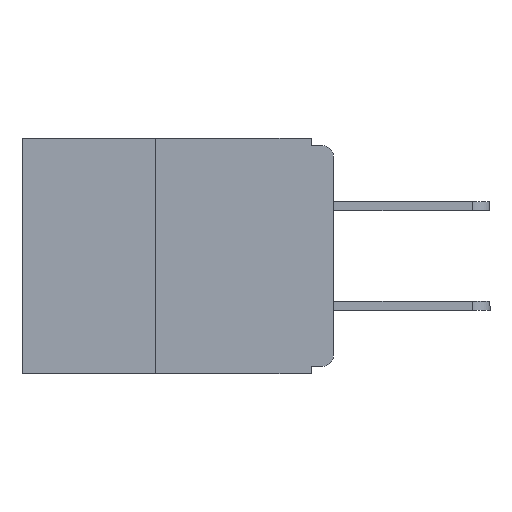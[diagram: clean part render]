
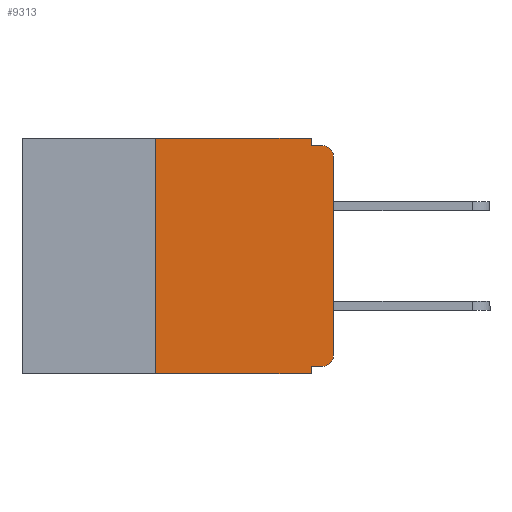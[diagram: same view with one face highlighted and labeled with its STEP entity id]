
A CAD part, left-side view. The second image highlights one B-rep face of the part: STEP entity #9313.
In plain terms, the highlighted planar face has unit normal (-1, 0, 0).
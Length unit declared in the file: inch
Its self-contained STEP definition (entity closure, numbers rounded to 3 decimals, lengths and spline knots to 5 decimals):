
#285 = VERTEX_POINT ( 'NONE', #8248 ) ;
#560 = VECTOR ( 'NONE', #4195, 39.37008 ) ;
#679 = DIRECTION ( 'NONE',  ( 0., 0., 1. ) ) ;
#684 = VERTEX_POINT ( 'NONE', #11078 ) ;
#914 = LINE ( 'NONE', #20379, #15717 ) ;
#1093 = VECTOR ( 'NONE', #679, 39.37008 ) ;
#1956 = DIRECTION ( 'NONE',  ( 1., 0., 0. ) ) ;
#2394 = DIRECTION ( 'NONE',  ( -1., 0., 0. ) ) ;
#2707 = EDGE_CURVE ( 'NONE', #684, #4057, #21120, .T. ) ;
#3035 = CARTESIAN_POINT ( 'NONE',  ( 0., 0.25, 0. ) ) ;
#3144 = CARTESIAN_POINT ( 'NONE',  ( 0., 0.031, -0.32 ) ) ;
#3458 = VERTEX_POINT ( 'NONE', #3035 ) ;
#3592 = PLANE ( 'NONE',  #4601 ) ;
#4008 = EDGE_LOOP ( 'NONE', ( #6687, #7054, #7076, #7227, #7481, #7824, #8143, #8163, #8323, #8462 ) ) ;
#4057 = VERTEX_POINT ( 'NONE', #13959 ) ;
#4117 = LINE ( 'NONE', #20929, #13785 ) ;
#4195 = DIRECTION ( 'NONE',  ( 0., 1., 0. ) ) ;
#4463 = CIRCLE ( 'NONE', #12592, 0.015 ) ;
#4500 = AXIS2_PLACEMENT_3D ( 'NONE', #12736, #2394, #14424 ) ;
#4601 = AXIS2_PLACEMENT_3D ( 'NONE', #5316, #1956, #21097 ) ;
#4613 = DIRECTION ( 'NONE',  ( -1., 0., 0. ) ) ;
#4679 = LINE ( 'NONE', #7680, #560 ) ;
#5316 = CARTESIAN_POINT ( 'NONE',  ( 0., 0.437, 0. ) ) ;
#5976 = VECTOR ( 'NONE', #12562, 39.37008 ) ;
#6687 = ORIENTED_EDGE ( 'NONE', *, *, #2707, .T. ) ;
#7054 = ORIENTED_EDGE ( 'NONE', *, *, #12635, .T. ) ;
#7076 = ORIENTED_EDGE ( 'NONE', *, *, #15427, .F. ) ;
#7227 = ORIENTED_EDGE ( 'NONE', *, *, #19667, .F. ) ;
#7481 = ORIENTED_EDGE ( 'NONE', *, *, #15186, .F. ) ;
#7680 = CARTESIAN_POINT ( 'NONE',  ( 0., 0., -0.32 ) ) ;
#7824 = ORIENTED_EDGE ( 'NONE', *, *, #20200, .F. ) ;
#8143 = ORIENTED_EDGE ( 'NONE', *, *, #9243, .T. ) ;
#8163 = ORIENTED_EDGE ( 'NONE', *, *, #12153, .F. ) ;
#8248 = CARTESIAN_POINT ( 'NONE',  ( 0., 0.015, -0.32 ) ) ;
#8323 = ORIENTED_EDGE ( 'NONE', *, *, #13721, .F. ) ;
#8462 = ORIENTED_EDGE ( 'NONE', *, *, #18484, .T. ) ;
#9059 = VERTEX_POINT ( 'NONE', #9771 ) ;
#9243 = EDGE_CURVE ( 'NONE', #19841, #9059, #17347, .T. ) ;
#9313 = ADVANCED_FACE ( 'NONE', ( #15789 ), #3592, .F. ) ;
#9710 = VECTOR ( 'NONE', #11576, 39.37008 ) ;
#9771 = CARTESIAN_POINT ( 'NONE',  ( 0., 0.031, -0.33 ) ) ;
#9897 = CARTESIAN_POINT ( 'NONE',  ( 0., 0.25, -0.33 ) ) ;
#10280 = LINE ( 'NONE', #14981, #9710 ) ;
#10506 = DIRECTION ( 'NONE',  ( 0., 0., -1. ) ) ;
#11077 = CARTESIAN_POINT ( 'NONE',  ( 0., 0.25, -0.33 ) ) ;
#11078 = CARTESIAN_POINT ( 'NONE',  ( 0., 0., -0.305 ) ) ;
#11576 = DIRECTION ( 'NONE',  ( 0., -1., 0. ) ) ;
#11728 = CARTESIAN_POINT ( 'NONE',  ( 0., 0.031, -0.01 ) ) ;
#12050 = CARTESIAN_POINT ( 'NONE',  ( 0., 0.437, -0.33 ) ) ;
#12153 = EDGE_CURVE ( 'NONE', #13985, #9059, #914, .T. ) ;
#12394 = VECTOR ( 'NONE', #21796, 39.37008 ) ;
#12462 = VECTOR ( 'NONE', #16134, 39.37008 ) ;
#12562 = DIRECTION ( 'NONE',  ( 0., -1., 0. ) ) ;
#12592 = AXIS2_PLACEMENT_3D ( 'NONE', #14888, #4613, #16549 ) ;
#12635 = EDGE_CURVE ( 'NONE', #4057, #15922, #4463, .T. ) ;
#12736 = CARTESIAN_POINT ( 'NONE',  ( 0., 0.015, -0.305 ) ) ;
#12834 = DIRECTION ( 'NONE',  ( 0., 0., -1. ) ) ;
#13721 = EDGE_CURVE ( 'NONE', #285, #13985, #4679, .T. ) ;
#13785 = VECTOR ( 'NONE', #12834, 39.37008 ) ;
#13959 = CARTESIAN_POINT ( 'NONE',  ( 0., 0., -0.025 ) ) ;
#13985 = VERTEX_POINT ( 'NONE', #3144 ) ;
#13996 = VERTEX_POINT ( 'NONE', #11728 ) ;
#14324 = LINE ( 'NONE', #11077, #1093 ) ;
#14424 = DIRECTION ( 'NONE',  ( 0., 0., -1. ) ) ;
#14888 = CARTESIAN_POINT ( 'NONE',  ( 0., 0.015, -0.025 ) ) ;
#14981 = CARTESIAN_POINT ( 'NONE',  ( 0., 0., -0.01 ) ) ;
#15186 = EDGE_CURVE ( 'NONE', #3458, #16018, #19866, .T. ) ;
#15427 = EDGE_CURVE ( 'NONE', #13996, #15922, #10280, .T. ) ;
#15717 = VECTOR ( 'NONE', #10506, 39.37008 ) ;
#15789 = FACE_OUTER_BOUND ( 'NONE', #4008, .T. ) ;
#15848 = CARTESIAN_POINT ( 'NONE',  ( 0., 0.437, 0. ) ) ;
#15922 = VERTEX_POINT ( 'NONE', #21063 ) ;
#16018 = VERTEX_POINT ( 'NONE', #18141 ) ;
#16134 = DIRECTION ( 'NONE',  ( 0., 0., 1. ) ) ;
#16153 = CARTESIAN_POINT ( 'NONE',  ( 0., 0., 0. ) ) ;
#16549 = DIRECTION ( 'NONE',  ( 0., 0., -1. ) ) ;
#17347 = LINE ( 'NONE', #12050, #12394 ) ;
#18141 = CARTESIAN_POINT ( 'NONE',  ( 0., 0.031, 0. ) ) ;
#18484 = EDGE_CURVE ( 'NONE', #285, #684, #20442, .T. ) ;
#19667 = EDGE_CURVE ( 'NONE', #16018, #13996, #4117, .T. ) ;
#19841 = VERTEX_POINT ( 'NONE', #9897 ) ;
#19866 = LINE ( 'NONE', #15848, #5976 ) ;
#20200 = EDGE_CURVE ( 'NONE', #19841, #3458, #14324, .T. ) ;
#20379 = CARTESIAN_POINT ( 'NONE',  ( 0., 0.031, -0.33 ) ) ;
#20442 = CIRCLE ( 'NONE', #4500, 0.015 ) ;
#20929 = CARTESIAN_POINT ( 'NONE',  ( 0., 0.031, 0. ) ) ;
#21063 = CARTESIAN_POINT ( 'NONE',  ( 0., 0.015, -0.01 ) ) ;
#21097 = DIRECTION ( 'NONE',  ( 0., 0., -1. ) ) ;
#21120 = LINE ( 'NONE', #16153, #12462 ) ;
#21796 = DIRECTION ( 'NONE',  ( 0., -1., 0. ) ) ;
